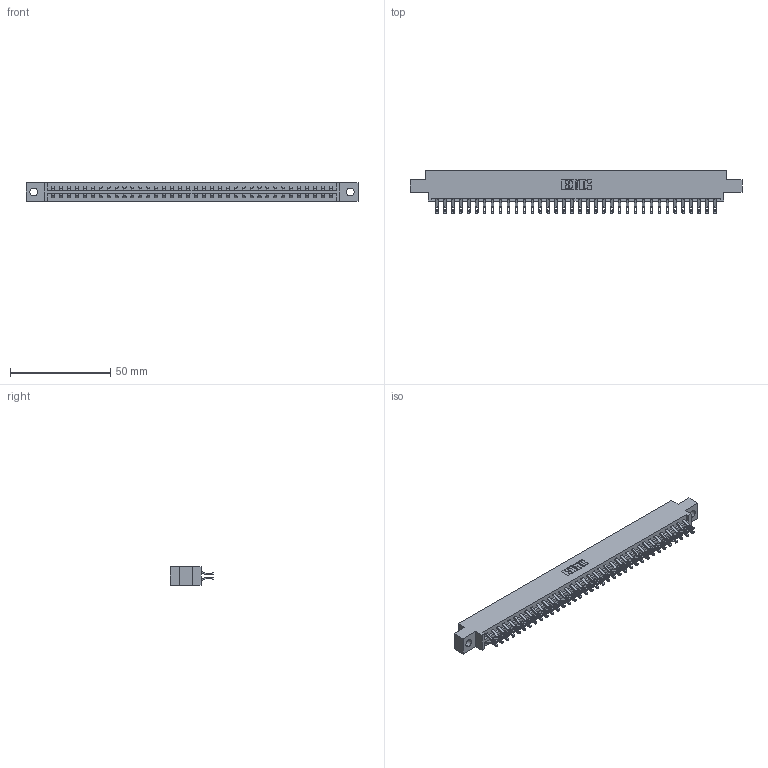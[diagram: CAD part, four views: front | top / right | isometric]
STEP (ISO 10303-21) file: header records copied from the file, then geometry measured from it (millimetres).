
FILE_DESCRIPTION (( 'STEP AP203' ), '1' );
FILE_NAME ('337-072-555-804.STEP', '2018-08-11T15:24:02', ( '' ), ( '' ), 'SwSTEP 2.0', 'SolidWorks 2016', '' );
FILE_SCHEMA (( 'CONFIG_CONTROL_DESIGN' ));
Length unit declared in the file: inch
Products named in the file (3): 337-072-555-804; 337 Part_0.170 Offset - 0.156 Dia-TH; 345-292-001_555 Tail
Assembly tree (73 placements, depth 2):
  337-072-555-804
    337 Part_0.170 Offset - 0.156 Dia-TH
    345-292-001_555 Tail  x72
Bounding box: 165.66 x 21.47 x 9.4 mm (x, y, z)
Volume: 17382 mm3; surface area: 20284.4 mm2
Topology: 73 solids, 73 shells, 4438 faces, 13931 edges, 9286 vertices
Faces by surface type: plane 2666, cylinder 1772
Entity records: 29149 total; most frequent: CARTESIAN_POINT 4952, ORIENTED_EDGE 4858, DIRECTION 4193, EDGE_CURVE 2429, VECTOR 2281, LINE 2281, VERTEX_POINT 1618, AXIS2_PLACEMENT_3D 956
